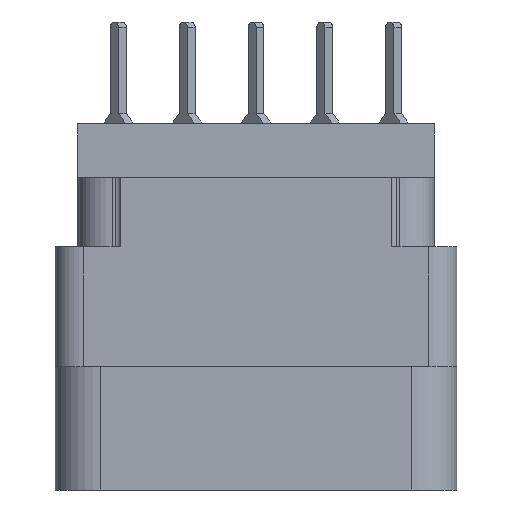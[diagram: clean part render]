
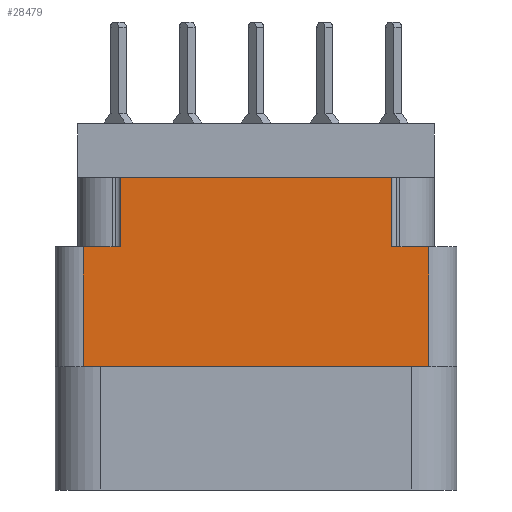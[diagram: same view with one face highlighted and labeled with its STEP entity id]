
A CAD part, left-side view. The second image highlights one B-rep face of the part: STEP entity #28479.
In plain terms, the highlighted planar face has unit normal (-1, 0, 0).
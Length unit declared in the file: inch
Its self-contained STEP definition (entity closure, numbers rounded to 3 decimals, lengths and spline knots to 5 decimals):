
#224 = LINE ( 'NONE', #12839, #1592 ) ;
#572 = DIRECTION ( 'NONE',  ( -1., 0., 0. ) ) ;
#1592 = VECTOR ( 'NONE', #26772, 39.37008 ) ;
#1983 = DIRECTION ( 'NONE',  ( 0., 0., 1. ) ) ;
#2239 = CARTESIAN_POINT ( 'NONE',  ( -1., -0.296, -0.268 ) ) ;
#2244 = LINE ( 'NONE', #10833, #19032 ) ;
#2473 = VECTOR ( 'NONE', #17883, 39.37008 ) ;
#2784 = CARTESIAN_POINT ( 'NONE',  ( -1., 0.438, -0.117 ) ) ;
#3062 = PLANE ( 'NONE',  #27266 ) ;
#4519 = CARTESIAN_POINT ( 'NONE',  ( -1., 0.376, -0.268 ) ) ;
#5602 = ORIENTED_EDGE ( 'NONE', *, *, #21748, .T. ) ;
#6351 = VECTOR ( 'NONE', #28826, 39.37008 ) ;
#7131 = VERTEX_POINT ( 'NONE', #27209 ) ;
#7534 = LINE ( 'NONE', #19795, #14582 ) ;
#8084 = DIRECTION ( 'NONE',  ( 0., -1., 0. ) ) ;
#8135 = LINE ( 'NONE', #2239, #36384 ) ;
#8208 = CARTESIAN_POINT ( 'NONE',  ( -1., 0.438, -0.268 ) ) ;
#9780 = VERTEX_POINT ( 'NONE', #4519 ) ;
#9946 = EDGE_CURVE ( 'NONE', #34242, #9780, #7534, .T. ) ;
#10019 = ORIENTED_EDGE ( 'NONE', *, *, #29024, .F. ) ;
#10833 = CARTESIAN_POINT ( 'NONE',  ( -1., -0.296, -0.268 ) ) ;
#11236 = DIRECTION ( 'NONE',  ( 0., 0., 1. ) ) ;
#11425 = DIRECTION ( 'NONE',  ( 0., 0., 1. ) ) ;
#11480 = CARTESIAN_POINT ( 'NONE',  ( -1., -0.376, -0.798 ) ) ;
#11718 = DIRECTION ( 'NONE',  ( 0., 0., 1. ) ) ;
#12804 = EDGE_CURVE ( 'NONE', #21648, #20800, #36521, .T. ) ;
#12839 = CARTESIAN_POINT ( 'NONE',  ( -1., 0.296, -0.268 ) ) ;
#13351 = EDGE_CURVE ( 'NONE', #7131, #21648, #224, .T. ) ;
#14123 = VERTEX_POINT ( 'NONE', #30427 ) ;
#14502 = EDGE_LOOP ( 'NONE', ( #26008, #5602, #27903, #30907, #27293, #23259, #18755, #10019 ) ) ;
#14582 = VECTOR ( 'NONE', #11425, 39.37008 ) ;
#14786 = FACE_OUTER_BOUND ( 'NONE', #14502, .T. ) ;
#16019 = LINE ( 'NONE', #33663, #31065 ) ;
#16629 = VERTEX_POINT ( 'NONE', #27915 ) ;
#17883 = DIRECTION ( 'NONE',  ( 0., -1., 0. ) ) ;
#18755 = ORIENTED_EDGE ( 'NONE', *, *, #13351, .F. ) ;
#18935 = EDGE_CURVE ( 'NONE', #16629, #20800, #8135, .T. ) ;
#19032 = VECTOR ( 'NONE', #8084, 39.37008 ) ;
#19795 = CARTESIAN_POINT ( 'NONE',  ( -1., 0.376, -0.798 ) ) ;
#20384 = CARTESIAN_POINT ( 'NONE',  ( -1., 0.296, -0.117 ) ) ;
#20800 = VERTEX_POINT ( 'NONE', #30937 ) ;
#21455 = CARTESIAN_POINT ( 'NONE',  ( -1., -0.376, -0.268 ) ) ;
#21507 = LINE ( 'NONE', #23698, #2473 ) ;
#21648 = VERTEX_POINT ( 'NONE', #20384 ) ;
#21748 = EDGE_CURVE ( 'NONE', #34242, #14123, #21507, .T. ) ;
#23259 = ORIENTED_EDGE ( 'NONE', *, *, #12804, .F. ) ;
#23698 = CARTESIAN_POINT ( 'NONE',  ( -1., 0., -0.529 ) ) ;
#24418 = EDGE_CURVE ( 'NONE', #14123, #25544, #16019, .T. ) ;
#25544 = VERTEX_POINT ( 'NONE', #21455 ) ;
#25756 = EDGE_CURVE ( 'NONE', #16629, #25544, #2244, .T. ) ;
#26008 = ORIENTED_EDGE ( 'NONE', *, *, #9946, .F. ) ;
#26772 = DIRECTION ( 'NONE',  ( 0., 0., 1. ) ) ;
#27209 = CARTESIAN_POINT ( 'NONE',  ( -1., 0.296, -0.268 ) ) ;
#27266 = AXIS2_PLACEMENT_3D ( 'NONE', #11480, #572, #11718 ) ;
#27293 = ORIENTED_EDGE ( 'NONE', *, *, #18935, .T. ) ;
#27903 = ORIENTED_EDGE ( 'NONE', *, *, #24418, .T. ) ;
#27915 = CARTESIAN_POINT ( 'NONE',  ( -1., -0.296, -0.268 ) ) ;
#28479 = ADVANCED_FACE ( 'NONE', ( #14786 ), #3062, .T. ) ;
#28826 = DIRECTION ( 'NONE',  ( 0., -1., 0. ) ) ;
#29024 = EDGE_CURVE ( 'NONE', #9780, #7131, #31115, .T. ) ;
#30427 = CARTESIAN_POINT ( 'NONE',  ( -1., -0.376, -0.529 ) ) ;
#30907 = ORIENTED_EDGE ( 'NONE', *, *, #25756, .F. ) ;
#30937 = CARTESIAN_POINT ( 'NONE',  ( -1., -0.296, -0.117 ) ) ;
#31065 = VECTOR ( 'NONE', #11236, 39.37008 ) ;
#31115 = LINE ( 'NONE', #8208, #6351 ) ;
#33400 = DIRECTION ( 'NONE',  ( 0., -1., 0. ) ) ;
#33663 = CARTESIAN_POINT ( 'NONE',  ( -1., -0.376, -0.798 ) ) ;
#34242 = VERTEX_POINT ( 'NONE', #35459 ) ;
#34761 = VECTOR ( 'NONE', #33400, 39.37008 ) ;
#35459 = CARTESIAN_POINT ( 'NONE',  ( -1., 0.376, -0.529 ) ) ;
#36384 = VECTOR ( 'NONE', #1983, 39.37008 ) ;
#36521 = LINE ( 'NONE', #2784, #34761 ) ;
